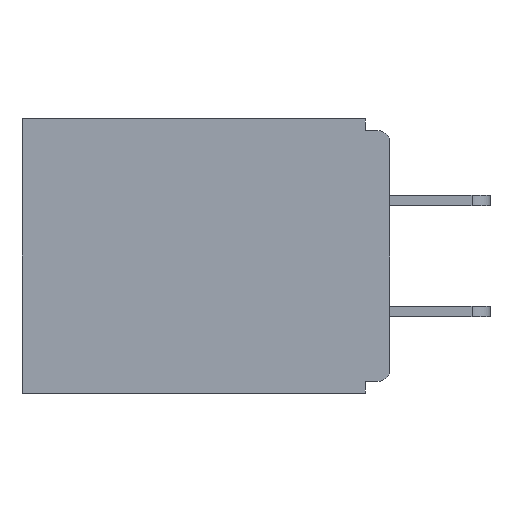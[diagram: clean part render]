
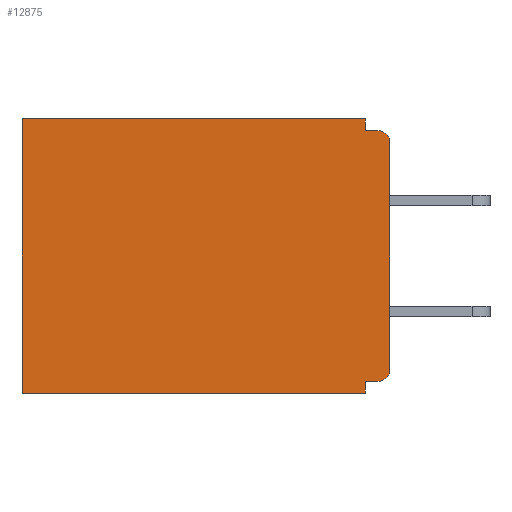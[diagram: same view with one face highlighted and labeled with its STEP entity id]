
A CAD part, left-side view. The second image highlights one B-rep face of the part: STEP entity #12875.
In plain terms, the highlighted planar face has unit normal (-1, 0, 0).
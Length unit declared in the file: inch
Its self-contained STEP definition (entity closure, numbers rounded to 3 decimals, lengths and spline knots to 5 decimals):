
#30 = DIRECTION ( 'NONE',  ( 0., -1., 0. ) ) ;
#42 = AXIS2_PLACEMENT_3D ( 'NONE', #11917, #1225, #12893 ) ;
#53 = ORIENTED_EDGE ( 'NONE', *, *, #7617, .F. ) ;
#183 = CIRCLE ( 'NONE', #42, 0.015 ) ;
#222 = CARTESIAN_POINT ( 'NONE',  ( 0.298, 0.031, -0.015 ) ) ;
#484 = ORIENTED_EDGE ( 'NONE', *, *, #11288, .F. ) ;
#832 = VERTEX_POINT ( 'NONE', #919 ) ;
#890 = CARTESIAN_POINT ( 'NONE',  ( 0.298, 0.46, -0.343 ) ) ;
#897 = VECTOR ( 'NONE', #3337, 39.37008 ) ;
#919 = CARTESIAN_POINT ( 'NONE',  ( 0.298, 0.46, 0. ) ) ;
#1225 = DIRECTION ( 'NONE',  ( -1., 0., 0. ) ) ;
#1308 = VERTEX_POINT ( 'NONE', #13911 ) ;
#1322 = EDGE_CURVE ( 'NONE', #2321, #832, #14196, .T. ) ;
#1586 = PLANE ( 'NONE',  #11757 ) ;
#2150 = VECTOR ( 'NONE', #7047, 39.37008 ) ;
#2321 = VERTEX_POINT ( 'NONE', #12424 ) ;
#2513 = VECTOR ( 'NONE', #4577, 39.37008 ) ;
#3211 = VERTEX_POINT ( 'NONE', #5140 ) ;
#3333 = VECTOR ( 'NONE', #15104, 39.37008 ) ;
#3337 = DIRECTION ( 'NONE',  ( 0., 1., 0. ) ) ;
#3405 = CARTESIAN_POINT ( 'NONE',  ( 0.298, 0.031, -0.343 ) ) ;
#3429 = VERTEX_POINT ( 'NONE', #890 ) ;
#3715 = LINE ( 'NONE', #11661, #3333 ) ;
#4005 = DIRECTION ( 'NONE',  ( 0., 0., -1. ) ) ;
#4118 = VECTOR ( 'NONE', #6682, 39.37008 ) ;
#4416 = CARTESIAN_POINT ( 'NONE',  ( 0.298, 0.46, 0. ) ) ;
#4577 = DIRECTION ( 'NONE',  ( 0., 1., 0. ) ) ;
#4706 = ORIENTED_EDGE ( 'NONE', *, *, #11290, .F. ) ;
#5140 = CARTESIAN_POINT ( 'NONE',  ( 0.298, 0.015, -0.328 ) ) ;
#5148 = LINE ( 'NONE', #12929, #15124 ) ;
#5496 = LINE ( 'NONE', #12825, #2150 ) ;
#5671 = DIRECTION ( 'NONE',  ( 0., 0., -1. ) ) ;
#6682 = DIRECTION ( 'NONE',  ( 0., 0., -1. ) ) ;
#6761 = ORIENTED_EDGE ( 'NONE', *, *, #7935, .T. ) ;
#7047 = DIRECTION ( 'NONE',  ( 0., 0., -1. ) ) ;
#7466 = VERTEX_POINT ( 'NONE', #3405 ) ;
#7499 = LINE ( 'NONE', #7851, #13190 ) ;
#7588 = CARTESIAN_POINT ( 'NONE',  ( 0.298, 0.015, -0.313 ) ) ;
#7617 = EDGE_CURVE ( 'NONE', #1308, #7466, #11642, .T. ) ;
#7650 = ORIENTED_EDGE ( 'NONE', *, *, #13862, .T. ) ;
#7662 = EDGE_CURVE ( 'NONE', #11919, #11721, #3715, .T. ) ;
#7680 = EDGE_CURVE ( 'NONE', #11919, #11822, #183, .T. ) ;
#7851 = CARTESIAN_POINT ( 'NONE',  ( 0.298, 0., -0.328 ) ) ;
#7935 = EDGE_CURVE ( 'NONE', #3211, #11721, #8148, .T. ) ;
#8103 = EDGE_CURVE ( 'NONE', #9528, #11822, #5148, .T. ) ;
#8148 = CIRCLE ( 'NONE', #10648, 0.015 ) ;
#8686 = ORIENTED_EDGE ( 'NONE', *, *, #7680, .T. ) ;
#8895 = VECTOR ( 'NONE', #5671, 39.37008 ) ;
#9528 = VERTEX_POINT ( 'NONE', #222 ) ;
#9781 = DIRECTION ( 'NONE',  ( 1., 0., 0. ) ) ;
#10485 = CARTESIAN_POINT ( 'NONE',  ( 0.298, 0., 0. ) ) ;
#10648 = AXIS2_PLACEMENT_3D ( 'NONE', #7588, #11135, #12265 ) ;
#10787 = ORIENTED_EDGE ( 'NONE', *, *, #12297, .F. ) ;
#10936 = LINE ( 'NONE', #4416, #4118 ) ;
#11135 = DIRECTION ( 'NONE',  ( -1., 0., 0. ) ) ;
#11288 = EDGE_CURVE ( 'NONE', #7466, #3429, #11768, .T. ) ;
#11290 = EDGE_CURVE ( 'NONE', #2321, #9528, #5496, .T. ) ;
#11379 = ORIENTED_EDGE ( 'NONE', *, *, #1322, .T. ) ;
#11557 = CARTESIAN_POINT ( 'NONE',  ( 0.298, 0.031, -0.343 ) ) ;
#11627 = CARTESIAN_POINT ( 'NONE',  ( 0.298, 0., -0.343 ) ) ;
#11642 = LINE ( 'NONE', #11557, #8895 ) ;
#11661 = CARTESIAN_POINT ( 'NONE',  ( 0.298, 0., 0. ) ) ;
#11721 = VERTEX_POINT ( 'NONE', #14215 ) ;
#11757 = AXIS2_PLACEMENT_3D ( 'NONE', #12091, #9781, #4005 ) ;
#11768 = LINE ( 'NONE', #11627, #2513 ) ;
#11822 = VERTEX_POINT ( 'NONE', #11911 ) ;
#11911 = CARTESIAN_POINT ( 'NONE',  ( 0.298, 0.015, -0.015 ) ) ;
#11917 = CARTESIAN_POINT ( 'NONE',  ( 0.298, 0.015, -0.03 ) ) ;
#11919 = VERTEX_POINT ( 'NONE', #14695 ) ;
#12091 = CARTESIAN_POINT ( 'NONE',  ( 0.298, 0., 0. ) ) ;
#12256 = FACE_OUTER_BOUND ( 'NONE', #14605, .T. ) ;
#12265 = DIRECTION ( 'NONE',  ( 0., 0., -1. ) ) ;
#12297 = EDGE_CURVE ( 'NONE', #3211, #1308, #7499, .T. ) ;
#12424 = CARTESIAN_POINT ( 'NONE',  ( 0.298, 0.031, 0. ) ) ;
#12613 = ORIENTED_EDGE ( 'NONE', *, *, #8103, .F. ) ;
#12825 = CARTESIAN_POINT ( 'NONE',  ( 0.298, 0.031, -0.343 ) ) ;
#12875 = ADVANCED_FACE ( 'NONE', ( #12256 ), #1586, .F. ) ;
#12893 = DIRECTION ( 'NONE',  ( 0., 0., -1. ) ) ;
#12929 = CARTESIAN_POINT ( 'NONE',  ( 0.298, 0., -0.015 ) ) ;
#13117 = ORIENTED_EDGE ( 'NONE', *, *, #7662, .F. ) ;
#13190 = VECTOR ( 'NONE', #13803, 39.37008 ) ;
#13803 = DIRECTION ( 'NONE',  ( 0., 1., 0. ) ) ;
#13862 = EDGE_CURVE ( 'NONE', #832, #3429, #10936, .T. ) ;
#13911 = CARTESIAN_POINT ( 'NONE',  ( 0.298, 0.031, -0.328 ) ) ;
#14196 = LINE ( 'NONE', #10485, #897 ) ;
#14215 = CARTESIAN_POINT ( 'NONE',  ( 0.298, 0., -0.313 ) ) ;
#14605 = EDGE_LOOP ( 'NONE', ( #8686, #12613, #4706, #11379, #7650, #484, #53, #10787, #6761, #13117 ) ) ;
#14695 = CARTESIAN_POINT ( 'NONE',  ( 0.298, 0., -0.03 ) ) ;
#15104 = DIRECTION ( 'NONE',  ( 0., 0., -1. ) ) ;
#15124 = VECTOR ( 'NONE', #30, 39.37008 ) ;
